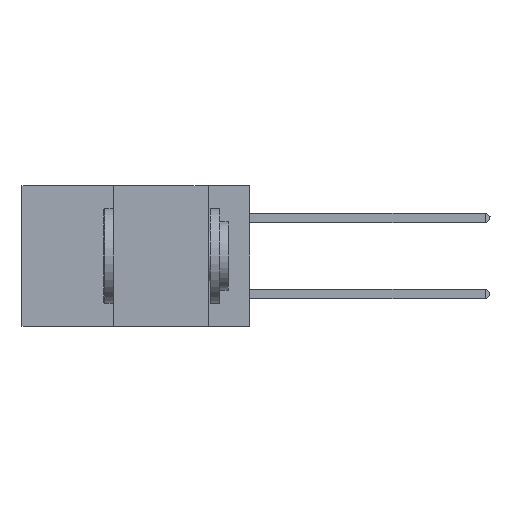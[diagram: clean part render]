
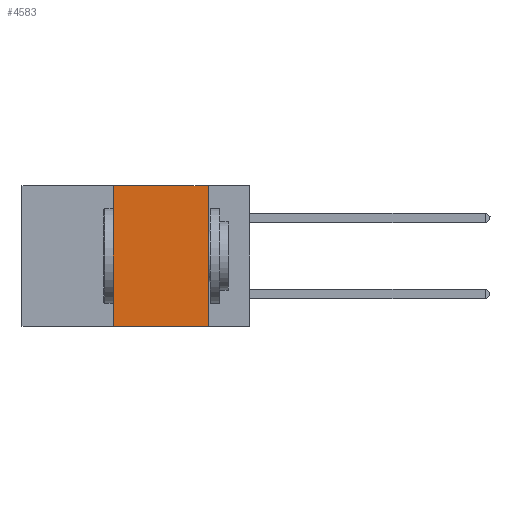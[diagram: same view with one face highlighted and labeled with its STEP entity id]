
A CAD part, left-side view. The second image highlights one B-rep face of the part: STEP entity #4583.
In plain terms, the highlighted planar face has unit normal (-1, 0, 0).
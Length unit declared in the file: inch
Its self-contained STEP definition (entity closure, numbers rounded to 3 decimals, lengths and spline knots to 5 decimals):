
#73 = DIRECTION ( 'NONE',  ( 0., 0., 1. ) ) ;
#444 = VECTOR ( 'NONE', #10762, 39.37008 ) ;
#987 = LINE ( 'NONE', #10359, #10042 ) ;
#1803 = VECTOR ( 'NONE', #3781, 39.37008 ) ;
#2061 = DIRECTION ( 'NONE',  ( 0., 0., -1. ) ) ;
#2146 = VERTEX_POINT ( 'NONE', #6694 ) ;
#2302 = CARTESIAN_POINT ( 'NONE',  ( 0., 0.11, 0. ) ) ;
#2532 = EDGE_LOOP ( 'NONE', ( #6667, #7809, #10020, #3897 ) ) ;
#2997 = AXIS2_PLACEMENT_3D ( 'NONE', #7945, #8820, #2061 ) ;
#3781 = DIRECTION ( 'NONE',  ( 0., 0., -1. ) ) ;
#3897 = ORIENTED_EDGE ( 'NONE', *, *, #9929, .T. ) ;
#4188 = EDGE_CURVE ( 'NONE', #4980, #2146, #10707, .T. ) ;
#4583 = ADVANCED_FACE ( 'NONE', ( #8670 ), #10517, .F. ) ;
#4980 = VERTEX_POINT ( 'NONE', #2302 ) ;
#5469 = VERTEX_POINT ( 'NONE', #9203 ) ;
#5752 = VECTOR ( 'NONE', #7720, 39.37008 ) ;
#6035 = EDGE_CURVE ( 'NONE', #6856, #5469, #987, .T. ) ;
#6102 = CARTESIAN_POINT ( 'NONE',  ( 0., 0.6, -0.37 ) ) ;
#6667 = ORIENTED_EDGE ( 'NONE', *, *, #4188, .F. ) ;
#6694 = CARTESIAN_POINT ( 'NONE',  ( 0., 0.11, -0.37 ) ) ;
#6856 = VERTEX_POINT ( 'NONE', #8580 ) ;
#7126 = EDGE_CURVE ( 'NONE', #5469, #4980, #10701, .T. ) ;
#7621 = CARTESIAN_POINT ( 'NONE',  ( 0., 0.6, 0. ) ) ;
#7720 = DIRECTION ( 'NONE',  ( 0., -1., 0. ) ) ;
#7809 = ORIENTED_EDGE ( 'NONE', *, *, #7126, .F. ) ;
#7945 = CARTESIAN_POINT ( 'NONE',  ( 0., 0.6, 0. ) ) ;
#8580 = CARTESIAN_POINT ( 'NONE',  ( 0., 0.36, -0.37 ) ) ;
#8670 = FACE_OUTER_BOUND ( 'NONE', #2532, .T. ) ;
#8808 = CARTESIAN_POINT ( 'NONE',  ( 0., 0.11, 0. ) ) ;
#8820 = DIRECTION ( 'NONE',  ( 1., 0., 0. ) ) ;
#9203 = CARTESIAN_POINT ( 'NONE',  ( 0., 0.36, 0. ) ) ;
#9453 = LINE ( 'NONE', #6102, #5752 ) ;
#9929 = EDGE_CURVE ( 'NONE', #6856, #2146, #9453, .T. ) ;
#10020 = ORIENTED_EDGE ( 'NONE', *, *, #6035, .F. ) ;
#10042 = VECTOR ( 'NONE', #73, 39.37008 ) ;
#10359 = CARTESIAN_POINT ( 'NONE',  ( 0., 0.36, 0. ) ) ;
#10517 = PLANE ( 'NONE',  #2997 ) ;
#10701 = LINE ( 'NONE', #7621, #444 ) ;
#10707 = LINE ( 'NONE', #8808, #1803 ) ;
#10762 = DIRECTION ( 'NONE',  ( 0., -1., 0. ) ) ;
